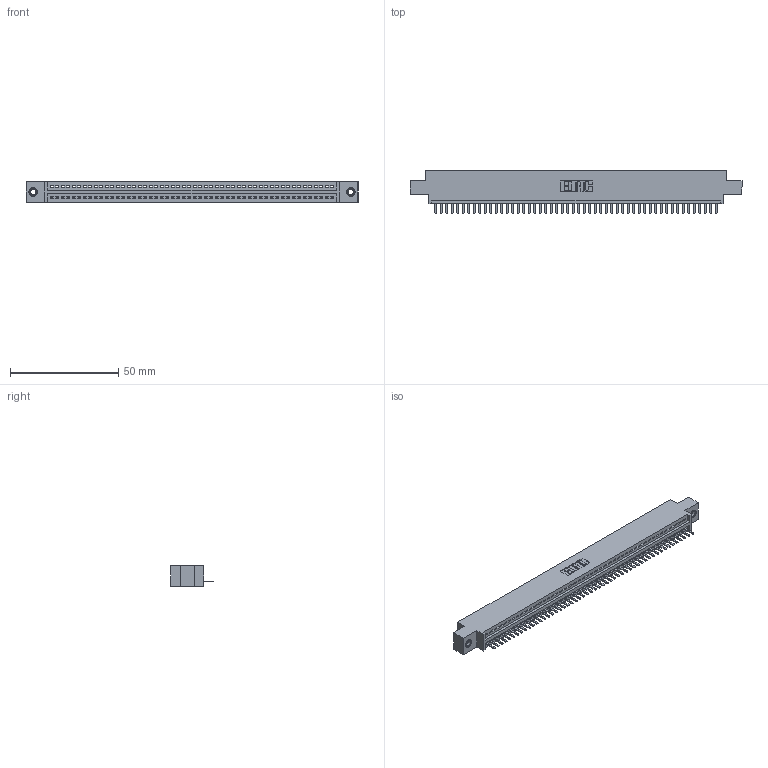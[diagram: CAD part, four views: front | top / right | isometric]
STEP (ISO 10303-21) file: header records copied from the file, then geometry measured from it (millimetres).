
FILE_DESCRIPTION (( 'STEP AP203' ), '1' );
FILE_NAME ('395-052-520-607.STEP', '2018-11-20T20:58:53', ( '' ), ( '' ), 'SwSTEP 2.0', 'SolidWorks 2016', '' );
FILE_SCHEMA (( 'CONFIG_CONTROL_DESIGN' ));
Length unit declared in the file: inch
Products named in the file (4): 345-292-001_345-293-120; 345 Part_0.170 Offset - 0.156 Dia-TI; 345-250-001_345-250-005-103; 395-052-520-607
Assembly tree (55 placements, depth 2):
  395-052-520-607
    345 Part_0.170 Offset - 0.156 Dia-TI
    345-292-001_345-293-120  x52
    345-250-001_345-250-005-103  x2
Bounding box: 153.29 x 19.68 x 9.4 mm (x, y, z)
Volume: 14365 mm3; surface area: 18895.4 mm2
Topology: 55 solids, 55 shells, 3414 faces, 10057 edges, 6558 vertices
Faces by surface type: plane 2300, cylinder 1098, cone 12, torus 4
Entity records: 39222 total; most frequent: CARTESIAN_POINT 6787, ORIENTED_EDGE 6754, DIRECTION 5927, EDGE_CURVE 3377, LINE 3013, VECTOR 3013, VERTEX_POINT 2244, AXIS2_PLACEMENT_3D 1457
